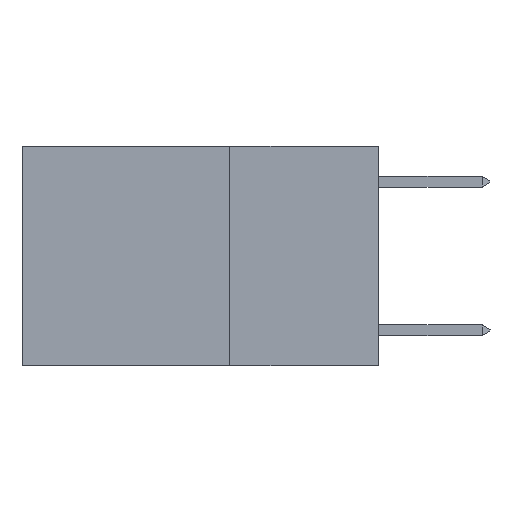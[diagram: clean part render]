
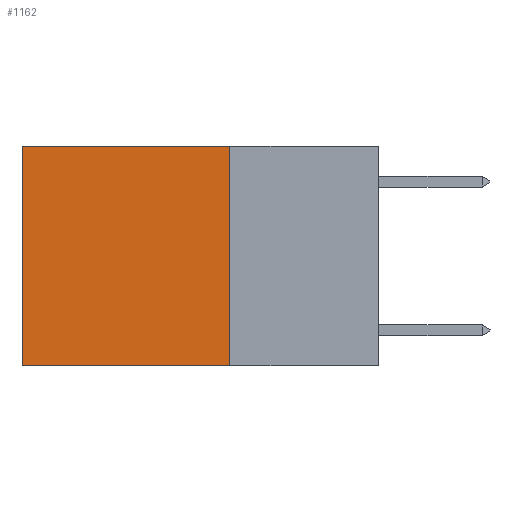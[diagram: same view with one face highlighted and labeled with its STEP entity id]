
A CAD part, left-side view. The second image highlights one B-rep face of the part: STEP entity #1162.
In plain terms, the highlighted planar face has unit normal (-1, 0, 0).
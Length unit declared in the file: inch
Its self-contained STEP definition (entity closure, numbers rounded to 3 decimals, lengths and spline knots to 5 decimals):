
#592 = DIRECTION ( 'NONE',  ( 0., 0., -1. ) ) ;
#1162 = ADVANCED_FACE ( 'NONE', ( #16322 ), #16663, .F. ) ;
#1387 = DIRECTION ( 'NONE',  ( 0., 0., -1. ) ) ;
#1895 = DIRECTION ( 'NONE',  ( 0., 1., 0. ) ) ;
#1969 = LINE ( 'NONE', #7296, #13592 ) ;
#2705 = CARTESIAN_POINT ( 'NONE',  ( 0.2625, 0.25, 0. ) ) ;
#3803 = LINE ( 'NONE', #17667, #6455 ) ;
#4032 = CARTESIAN_POINT ( 'NONE',  ( 0.2625, 0.25, 0. ) ) ;
#5526 = DIRECTION ( 'NONE',  ( 1., 0., 0. ) ) ;
#5666 = CARTESIAN_POINT ( 'NONE',  ( 0.2625, 0.6, 0. ) ) ;
#6455 = VECTOR ( 'NONE', #12110, 39.37008 ) ;
#7215 = EDGE_CURVE ( 'NONE', #15488, #14660, #1969, .T. ) ;
#7296 = CARTESIAN_POINT ( 'NONE',  ( 0.2625, 0.25, -0.37 ) ) ;
#9310 = EDGE_CURVE ( 'NONE', #13840, #15488, #17507, .T. ) ;
#9552 = VERTEX_POINT ( 'NONE', #11634 ) ;
#10154 = VECTOR ( 'NONE', #1387, 39.37008 ) ;
#11559 = ORIENTED_EDGE ( 'NONE', *, *, #16986, .T. ) ;
#11634 = CARTESIAN_POINT ( 'NONE',  ( 0.2625, 0.6, 0. ) ) ;
#12110 = DIRECTION ( 'NONE',  ( 0., 1., 0. ) ) ;
#12373 = EDGE_LOOP ( 'NONE', ( #11559, #15445, #17761, #17223 ) ) ;
#12787 = LINE ( 'NONE', #5666, #10154 ) ;
#13592 = VECTOR ( 'NONE', #1895, 39.37008 ) ;
#13691 = AXIS2_PLACEMENT_3D ( 'NONE', #2705, #5526, #592 ) ;
#13728 = VECTOR ( 'NONE', #16713, 39.37008 ) ;
#13840 = VERTEX_POINT ( 'NONE', #18025 ) ;
#14252 = CARTESIAN_POINT ( 'NONE',  ( 0.2625, 0.6, -0.37 ) ) ;
#14660 = VERTEX_POINT ( 'NONE', #14252 ) ;
#15445 = ORIENTED_EDGE ( 'NONE', *, *, #7215, .F. ) ;
#15488 = VERTEX_POINT ( 'NONE', #17547 ) ;
#15719 = EDGE_CURVE ( 'NONE', #13840, #9552, #3803, .T. ) ;
#16322 = FACE_OUTER_BOUND ( 'NONE', #12373, .T. ) ;
#16663 = PLANE ( 'NONE',  #13691 ) ;
#16713 = DIRECTION ( 'NONE',  ( 0., 0., -1. ) ) ;
#16986 = EDGE_CURVE ( 'NONE', #9552, #14660, #12787, .T. ) ;
#17223 = ORIENTED_EDGE ( 'NONE', *, *, #15719, .T. ) ;
#17507 = LINE ( 'NONE', #4032, #13728 ) ;
#17547 = CARTESIAN_POINT ( 'NONE',  ( 0.2625, 0.25, -0.37 ) ) ;
#17667 = CARTESIAN_POINT ( 'NONE',  ( 0.2625, 0.25, 0. ) ) ;
#17761 = ORIENTED_EDGE ( 'NONE', *, *, #9310, .F. ) ;
#18025 = CARTESIAN_POINT ( 'NONE',  ( 0.2625, 0.25, 0. ) ) ;
